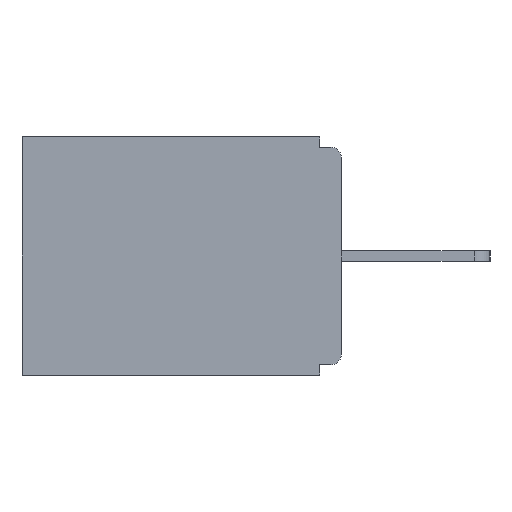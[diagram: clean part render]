
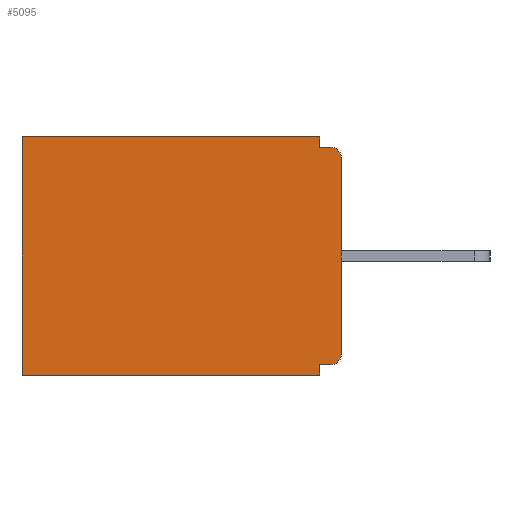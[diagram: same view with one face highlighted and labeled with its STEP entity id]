
A CAD part, left-side view. The second image highlights one B-rep face of the part: STEP entity #5095.
In plain terms, the highlighted planar face has unit normal (-1, 0, 0).
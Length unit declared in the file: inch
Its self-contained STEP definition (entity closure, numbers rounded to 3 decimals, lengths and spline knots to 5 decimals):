
#5 = LINE ( 'NONE', #2027, #1125 ) ;
#150 = DIRECTION ( 'NONE',  ( 0., 0., -1. ) ) ;
#207 = CARTESIAN_POINT ( 'NONE',  ( 0.298, 0., 0. ) ) ;
#273 = EDGE_CURVE ( 'NONE', #2963, #4913, #7524, .T. ) ;
#432 = DIRECTION ( 'NONE',  ( 0., 0., -1. ) ) ;
#990 = DIRECTION ( 'NONE',  ( 0., 1., 0. ) ) ;
#1006 = EDGE_CURVE ( 'NONE', #1532, #12374, #2347, .T. ) ;
#1125 = VECTOR ( 'NONE', #4090, 39.37008 ) ;
#1435 = ORIENTED_EDGE ( 'NONE', *, *, #5775, .F. ) ;
#1532 = VERTEX_POINT ( 'NONE', #2965 ) ;
#1845 = CARTESIAN_POINT ( 'NONE',  ( 0.298, 0.015, -0.313 ) ) ;
#1856 = CARTESIAN_POINT ( 'NONE',  ( 0.298, 0., -0.015 ) ) ;
#2027 = CARTESIAN_POINT ( 'NONE',  ( 0.298, 0., 0. ) ) ;
#2318 = DIRECTION ( 'NONE',  ( -1., 0., 0. ) ) ;
#2327 = EDGE_CURVE ( 'NONE', #5214, #5508, #7637, .T. ) ;
#2347 = LINE ( 'NONE', #6299, #2541 ) ;
#2418 = CIRCLE ( 'NONE', #3904, 0.015 ) ;
#2462 = CARTESIAN_POINT ( 'NONE',  ( 0.298, 0.015, -0.03 ) ) ;
#2475 = CARTESIAN_POINT ( 'NONE',  ( 0.298, 0., -0.328 ) ) ;
#2494 = CARTESIAN_POINT ( 'NONE',  ( 0.298, 0., -0.03 ) ) ;
#2541 = VECTOR ( 'NONE', #5327, 39.37008 ) ;
#2846 = VERTEX_POINT ( 'NONE', #3415 ) ;
#2899 = EDGE_CURVE ( 'NONE', #8500, #12374, #11658, .T. ) ;
#2963 = VERTEX_POINT ( 'NONE', #7457 ) ;
#2965 = CARTESIAN_POINT ( 'NONE',  ( 0.298, 0.031, -0.343 ) ) ;
#3230 = DIRECTION ( 'NONE',  ( 0., 0., -1. ) ) ;
#3415 = CARTESIAN_POINT ( 'NONE',  ( 0.298, 0., -0.313 ) ) ;
#3466 = AXIS2_PLACEMENT_3D ( 'NONE', #1845, #10025, #7041 ) ;
#3652 = EDGE_CURVE ( 'NONE', #5025, #5214, #6428, .T. ) ;
#3800 = VECTOR ( 'NONE', #990, 39.37008 ) ;
#3899 = CIRCLE ( 'NONE', #3466, 0.015 ) ;
#3904 = AXIS2_PLACEMENT_3D ( 'NONE', #2462, #2318, #432 ) ;
#4090 = DIRECTION ( 'NONE',  ( 0., 1., 0. ) ) ;
#4251 = DIRECTION ( 'NONE',  ( 1., 0., 0. ) ) ;
#4430 = CARTESIAN_POINT ( 'NONE',  ( 0.298, 0.031, -0.343 ) ) ;
#4913 = VERTEX_POINT ( 'NONE', #12227 ) ;
#5025 = VERTEX_POINT ( 'NONE', #7416 ) ;
#5095 = ADVANCED_FACE ( 'NONE', ( #9416 ), #8349, .F. ) ;
#5214 = VERTEX_POINT ( 'NONE', #11745 ) ;
#5327 = DIRECTION ( 'NONE',  ( 0., 1., 0. ) ) ;
#5352 = EDGE_CURVE ( 'NONE', #5025, #8500, #5, .T. ) ;
#5485 = ORIENTED_EDGE ( 'NONE', *, *, #2899, .T. ) ;
#5508 = VERTEX_POINT ( 'NONE', #12937 ) ;
#5775 = EDGE_CURVE ( 'NONE', #9697, #2846, #8475, .T. ) ;
#5877 = VECTOR ( 'NONE', #150, 39.37008 ) ;
#6224 = ORIENTED_EDGE ( 'NONE', *, *, #2327, .F. ) ;
#6268 = VECTOR ( 'NONE', #12665, 39.37008 ) ;
#6299 = CARTESIAN_POINT ( 'NONE',  ( 0.298, 0., -0.343 ) ) ;
#6428 = LINE ( 'NONE', #10409, #5877 ) ;
#6435 = CARTESIAN_POINT ( 'NONE',  ( 0.298, 0., 0. ) ) ;
#6641 = CARTESIAN_POINT ( 'NONE',  ( 0.298, 0.46, -0.343 ) ) ;
#7041 = DIRECTION ( 'NONE',  ( 0., 0., -1. ) ) ;
#7398 = CARTESIAN_POINT ( 'NONE',  ( 0.298, 0.46, 0. ) ) ;
#7416 = CARTESIAN_POINT ( 'NONE',  ( 0.298, 0.031, 0. ) ) ;
#7457 = CARTESIAN_POINT ( 'NONE',  ( 0.298, 0.015, -0.328 ) ) ;
#7524 = LINE ( 'NONE', #2475, #3800 ) ;
#7595 = EDGE_CURVE ( 'NONE', #4913, #1532, #10544, .T. ) ;
#7637 = LINE ( 'NONE', #1856, #11964 ) ;
#7894 = DIRECTION ( 'NONE',  ( 0., -1., 0. ) ) ;
#7988 = EDGE_LOOP ( 'NONE', ( #10665, #6224, #13078, #9763, #5485, #12470, #7991, #12885, #12918, #1435 ) ) ;
#7991 = ORIENTED_EDGE ( 'NONE', *, *, #7595, .F. ) ;
#8349 = PLANE ( 'NONE',  #10471 ) ;
#8475 = LINE ( 'NONE', #207, #11753 ) ;
#8500 = VERTEX_POINT ( 'NONE', #12362 ) ;
#8523 = DIRECTION ( 'NONE',  ( 0., 0., -1. ) ) ;
#8738 = VECTOR ( 'NONE', #8523, 39.37008 ) ;
#9228 = EDGE_CURVE ( 'NONE', #9697, #5508, #2418, .T. ) ;
#9416 = FACE_OUTER_BOUND ( 'NONE', #7988, .T. ) ;
#9697 = VERTEX_POINT ( 'NONE', #2494 ) ;
#9763 = ORIENTED_EDGE ( 'NONE', *, *, #5352, .T. ) ;
#10025 = DIRECTION ( 'NONE',  ( -1., 0., 0. ) ) ;
#10409 = CARTESIAN_POINT ( 'NONE',  ( 0.298, 0.031, -0.343 ) ) ;
#10471 = AXIS2_PLACEMENT_3D ( 'NONE', #6435, #4251, #10483 ) ;
#10483 = DIRECTION ( 'NONE',  ( 0., 0., -1. ) ) ;
#10544 = LINE ( 'NONE', #4430, #6268 ) ;
#10665 = ORIENTED_EDGE ( 'NONE', *, *, #9228, .T. ) ;
#11658 = LINE ( 'NONE', #7398, #8738 ) ;
#11745 = CARTESIAN_POINT ( 'NONE',  ( 0.298, 0.031, -0.015 ) ) ;
#11753 = VECTOR ( 'NONE', #3230, 39.37008 ) ;
#11964 = VECTOR ( 'NONE', #7894, 39.37008 ) ;
#12227 = CARTESIAN_POINT ( 'NONE',  ( 0.298, 0.031, -0.328 ) ) ;
#12362 = CARTESIAN_POINT ( 'NONE',  ( 0.298, 0.46, 0. ) ) ;
#12374 = VERTEX_POINT ( 'NONE', #6641 ) ;
#12470 = ORIENTED_EDGE ( 'NONE', *, *, #1006, .F. ) ;
#12507 = EDGE_CURVE ( 'NONE', #2963, #2846, #3899, .T. ) ;
#12665 = DIRECTION ( 'NONE',  ( 0., 0., -1. ) ) ;
#12885 = ORIENTED_EDGE ( 'NONE', *, *, #273, .F. ) ;
#12918 = ORIENTED_EDGE ( 'NONE', *, *, #12507, .T. ) ;
#12937 = CARTESIAN_POINT ( 'NONE',  ( 0.298, 0.015, -0.015 ) ) ;
#13078 = ORIENTED_EDGE ( 'NONE', *, *, #3652, .F. ) ;
